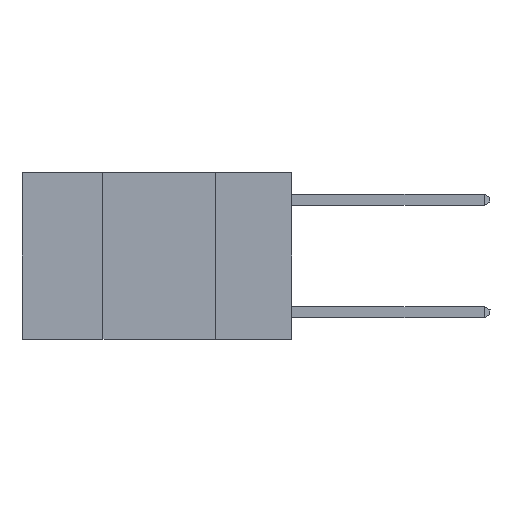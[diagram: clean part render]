
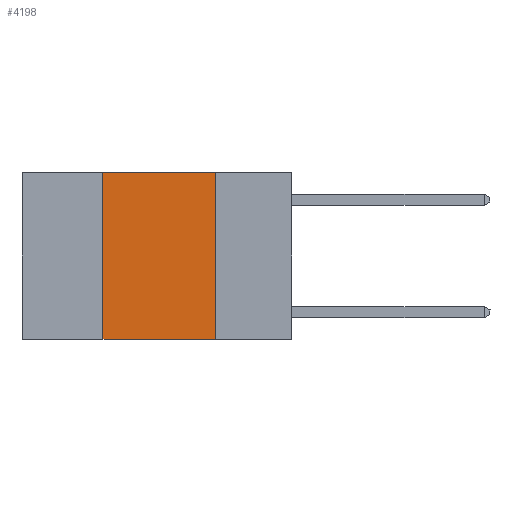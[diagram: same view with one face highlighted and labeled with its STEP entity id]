
A CAD part, left-side view. The second image highlights one B-rep face of the part: STEP entity #4198.
In plain terms, the highlighted planar face has unit normal (-1, 0, 0).
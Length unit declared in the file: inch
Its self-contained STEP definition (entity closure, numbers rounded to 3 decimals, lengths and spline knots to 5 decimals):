
#26 = CARTESIAN_POINT ( 'NONE',  ( 0., 0.42, 0. ) ) ;
#307 = VECTOR ( 'NONE', #3762, 39.37008 ) ;
#363 = DIRECTION ( 'NONE',  ( 0., 0., -1. ) ) ;
#542 = CARTESIAN_POINT ( 'NONE',  ( 0., 0.6, -0.37 ) ) ;
#548 = DIRECTION ( 'NONE',  ( 1., 0., 0. ) ) ;
#860 = CARTESIAN_POINT ( 'NONE',  ( 0., 0.6, 0. ) ) ;
#933 = PLANE ( 'NONE',  #8629 ) ;
#1051 = VERTEX_POINT ( 'NONE', #6755 ) ;
#1313 = VERTEX_POINT ( 'NONE', #2055 ) ;
#1385 = LINE ( 'NONE', #2039, #7516 ) ;
#1657 = VECTOR ( 'NONE', #2761, 39.37008 ) ;
#2039 = CARTESIAN_POINT ( 'NONE',  ( 0., 0.6, 0. ) ) ;
#2054 = ORIENTED_EDGE ( 'NONE', *, *, #7321, .F. ) ;
#2055 = CARTESIAN_POINT ( 'NONE',  ( 0., 0.17, 0. ) ) ;
#2454 = ORIENTED_EDGE ( 'NONE', *, *, #3717, .T. ) ;
#2497 = ORIENTED_EDGE ( 'NONE', *, *, #4619, .F. ) ;
#2539 = LINE ( 'NONE', #5373, #307 ) ;
#2696 = ORIENTED_EDGE ( 'NONE', *, *, #7395, .F. ) ;
#2761 = DIRECTION ( 'NONE',  ( 0., -1., 0. ) ) ;
#3562 = VECTOR ( 'NONE', #10202, 39.37008 ) ;
#3584 = LINE ( 'NONE', #542, #1657 ) ;
#3717 = EDGE_CURVE ( 'NONE', #7794, #6731, #3584, .T. ) ;
#3762 = DIRECTION ( 'NONE',  ( 0., 0., -1. ) ) ;
#3829 = LINE ( 'NONE', #26, #3562 ) ;
#4198 = ADVANCED_FACE ( 'NONE', ( #5454 ), #933, .F. ) ;
#4619 = EDGE_CURVE ( 'NONE', #7794, #1051, #3829, .T. ) ;
#5373 = CARTESIAN_POINT ( 'NONE',  ( 0., 0.17, 0. ) ) ;
#5454 = FACE_OUTER_BOUND ( 'NONE', #6923, .T. ) ;
#6058 = DIRECTION ( 'NONE',  ( 0., -1., 0. ) ) ;
#6731 = VERTEX_POINT ( 'NONE', #6815 ) ;
#6755 = CARTESIAN_POINT ( 'NONE',  ( 0., 0.42, 0. ) ) ;
#6815 = CARTESIAN_POINT ( 'NONE',  ( 0., 0.17, -0.37 ) ) ;
#6923 = EDGE_LOOP ( 'NONE', ( #2696, #2054, #2497, #2454 ) ) ;
#7321 = EDGE_CURVE ( 'NONE', #1051, #1313, #1385, .T. ) ;
#7395 = EDGE_CURVE ( 'NONE', #1313, #6731, #2539, .T. ) ;
#7466 = CARTESIAN_POINT ( 'NONE',  ( 0., 0.42, -0.37 ) ) ;
#7516 = VECTOR ( 'NONE', #6058, 39.37008 ) ;
#7794 = VERTEX_POINT ( 'NONE', #7466 ) ;
#8629 = AXIS2_PLACEMENT_3D ( 'NONE', #860, #548, #363 ) ;
#10202 = DIRECTION ( 'NONE',  ( 0., 0., 1. ) ) ;
